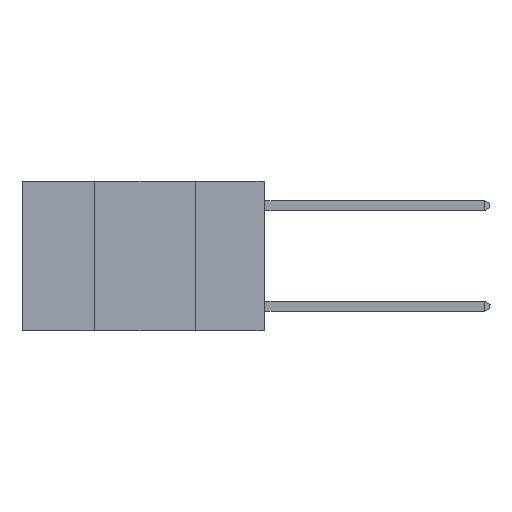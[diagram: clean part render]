
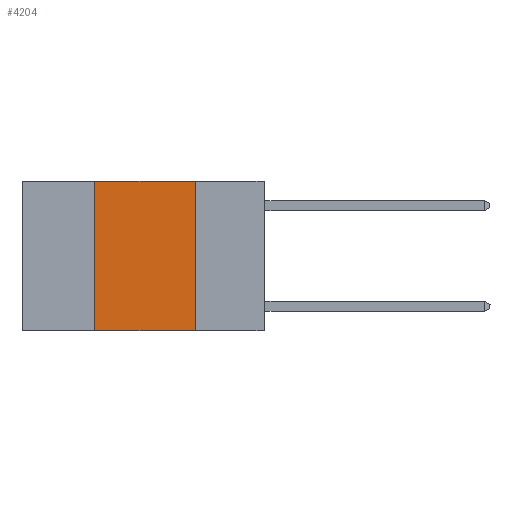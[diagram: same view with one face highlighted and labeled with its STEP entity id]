
A CAD part, left-side view. The second image highlights one B-rep face of the part: STEP entity #4204.
In plain terms, the highlighted planar face has unit normal (-1, 0, 0).
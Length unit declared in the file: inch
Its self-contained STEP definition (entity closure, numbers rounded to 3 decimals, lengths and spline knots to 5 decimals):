
#435 = DIRECTION ( 'NONE',  ( 1., 0., 0. ) ) ;
#487 = ORIENTED_EDGE ( 'NONE', *, *, #3090, .T. ) ;
#699 = CARTESIAN_POINT ( 'NONE',  ( 0., 0.42, 0. ) ) ;
#746 = CARTESIAN_POINT ( 'NONE',  ( 0., 0.17, 0. ) ) ;
#1143 = LINE ( 'NONE', #699, #11283 ) ;
#1792 = DIRECTION ( 'NONE',  ( 0., 0., -1. ) ) ;
#2685 = DIRECTION ( 'NONE',  ( 0., 0., 1. ) ) ;
#2804 = VERTEX_POINT ( 'NONE', #12424 ) ;
#2967 = CARTESIAN_POINT ( 'NONE',  ( 0., 0.42, -0.37 ) ) ;
#2974 = VECTOR ( 'NONE', #6930, 39.37008 ) ;
#3039 = VERTEX_POINT ( 'NONE', #7870 ) ;
#3090 = EDGE_CURVE ( 'NONE', #7426, #3039, #5944, .T. ) ;
#3331 = DIRECTION ( 'NONE',  ( 0., -1., 0. ) ) ;
#3333 = EDGE_LOOP ( 'NONE', ( #5423, #8068, #10653, #487 ) ) ;
#3418 = EDGE_CURVE ( 'NONE', #2804, #7877, #9475, .T. ) ;
#3501 = FACE_OUTER_BOUND ( 'NONE', #3333, .T. ) ;
#3647 = VECTOR ( 'NONE', #1792, 39.37008 ) ;
#3739 = EDGE_CURVE ( 'NONE', #7426, #2804, #1143, .T. ) ;
#4204 = ADVANCED_FACE ( 'NONE', ( #3501 ), #5343, .F. ) ;
#4313 = CARTESIAN_POINT ( 'NONE',  ( 0., 0.6, 0. ) ) ;
#4412 = EDGE_CURVE ( 'NONE', #7877, #3039, #8338, .T. ) ;
#4750 = CARTESIAN_POINT ( 'NONE',  ( 0., 0.17, 0. ) ) ;
#5343 = PLANE ( 'NONE',  #9409 ) ;
#5423 = ORIENTED_EDGE ( 'NONE', *, *, #4412, .F. ) ;
#5944 = LINE ( 'NONE', #8848, #2974 ) ;
#6930 = DIRECTION ( 'NONE',  ( 0., -1., 0. ) ) ;
#7353 = DIRECTION ( 'NONE',  ( 0., 0., -1. ) ) ;
#7426 = VERTEX_POINT ( 'NONE', #2967 ) ;
#7870 = CARTESIAN_POINT ( 'NONE',  ( 0., 0.17, -0.37 ) ) ;
#7877 = VERTEX_POINT ( 'NONE', #746 ) ;
#8068 = ORIENTED_EDGE ( 'NONE', *, *, #3418, .F. ) ;
#8338 = LINE ( 'NONE', #4750, #3647 ) ;
#8848 = CARTESIAN_POINT ( 'NONE',  ( 0., 0.6, -0.37 ) ) ;
#9175 = VECTOR ( 'NONE', #3331, 39.37008 ) ;
#9409 = AXIS2_PLACEMENT_3D ( 'NONE', #4313, #435, #7353 ) ;
#9475 = LINE ( 'NONE', #12175, #9175 ) ;
#10653 = ORIENTED_EDGE ( 'NONE', *, *, #3739, .F. ) ;
#11283 = VECTOR ( 'NONE', #2685, 39.37008 ) ;
#12175 = CARTESIAN_POINT ( 'NONE',  ( 0., 0.6, 0. ) ) ;
#12424 = CARTESIAN_POINT ( 'NONE',  ( 0., 0.42, 0. ) ) ;
